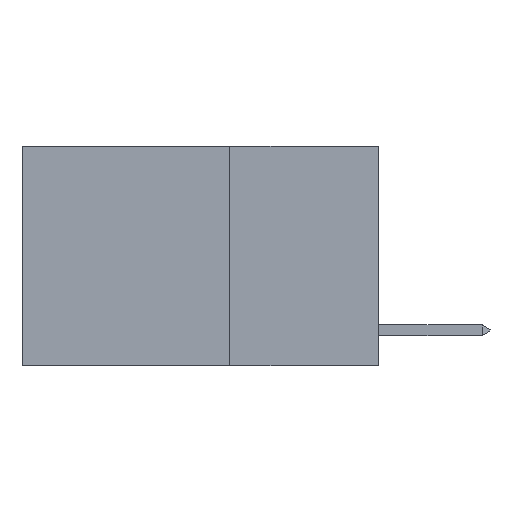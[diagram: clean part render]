
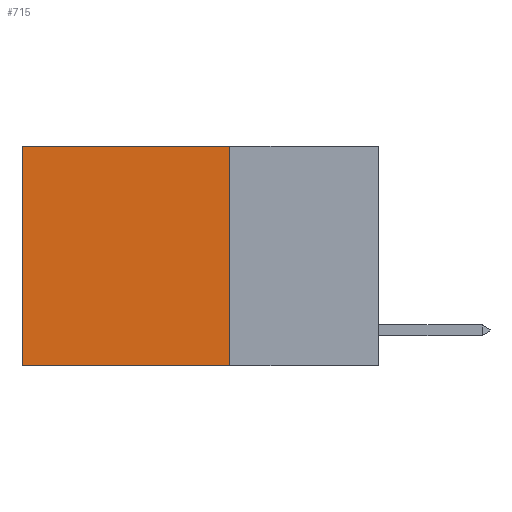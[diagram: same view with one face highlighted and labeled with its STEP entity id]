
A CAD part, left-side view. The second image highlights one B-rep face of the part: STEP entity #715.
In plain terms, the highlighted planar face has unit normal (-1, 0, 0).
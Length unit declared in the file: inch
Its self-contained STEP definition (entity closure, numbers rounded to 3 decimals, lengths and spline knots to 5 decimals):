
#715 = ADVANCED_FACE ( 'NONE', ( #7400 ), #13303, .F. ) ;
#927 = EDGE_CURVE ( 'NONE', #3811, #18361, #2249, .T. ) ;
#2249 = LINE ( 'NONE', #8657, #3781 ) ;
#3290 = LINE ( 'NONE', #7243, #19058 ) ;
#3325 = CARTESIAN_POINT ( 'NONE',  ( 0.2625, 0.25, -0.37 ) ) ;
#3564 = DIRECTION ( 'NONE',  ( 1., 0., 0. ) ) ;
#3781 = VECTOR ( 'NONE', #4310, 39.37008 ) ;
#3811 = VERTEX_POINT ( 'NONE', #4824 ) ;
#3913 = EDGE_CURVE ( 'NONE', #18361, #12568, #3290, .T. ) ;
#4310 = DIRECTION ( 'NONE',  ( 0., 1., 0. ) ) ;
#4824 = CARTESIAN_POINT ( 'NONE',  ( 0.2625, 0.25, 0. ) ) ;
#5467 = ORIENTED_EDGE ( 'NONE', *, *, #927, .T. ) ;
#7243 = CARTESIAN_POINT ( 'NONE',  ( 0.2625, 0.6, 0. ) ) ;
#7400 = FACE_OUTER_BOUND ( 'NONE', #17790, .T. ) ;
#7684 = CARTESIAN_POINT ( 'NONE',  ( 0.2625, 0.6, -0.37 ) ) ;
#8336 = EDGE_CURVE ( 'NONE', #3811, #10974, #24845, .T. ) ;
#8657 = CARTESIAN_POINT ( 'NONE',  ( 0.2625, 0.25, 0. ) ) ;
#8927 = ORIENTED_EDGE ( 'NONE', *, *, #8336, .F. ) ;
#10974 = VERTEX_POINT ( 'NONE', #3325 ) ;
#11381 = DIRECTION ( 'NONE',  ( 0., 0., -1. ) ) ;
#11484 = CARTESIAN_POINT ( 'NONE',  ( 0.2625, 0.25, 0. ) ) ;
#11681 = VECTOR ( 'NONE', #23865, 39.37008 ) ;
#11689 = ORIENTED_EDGE ( 'NONE', *, *, #14106, .F. ) ;
#12568 = VERTEX_POINT ( 'NONE', #7684 ) ;
#13303 = PLANE ( 'NONE',  #15225 ) ;
#13421 = DIRECTION ( 'NONE',  ( 0., 0., -1. ) ) ;
#14106 = EDGE_CURVE ( 'NONE', #10974, #12568, #16587, .T. ) ;
#15225 = AXIS2_PLACEMENT_3D ( 'NONE', #21033, #3564, #11381 ) ;
#16587 = LINE ( 'NONE', #20416, #11681 ) ;
#17790 = EDGE_LOOP ( 'NONE', ( #24351, #11689, #8927, #5467 ) ) ;
#18361 = VERTEX_POINT ( 'NONE', #24097 ) ;
#19058 = VECTOR ( 'NONE', #22681, 39.37008 ) ;
#20416 = CARTESIAN_POINT ( 'NONE',  ( 0.2625, 0.25, -0.37 ) ) ;
#21033 = CARTESIAN_POINT ( 'NONE',  ( 0.2625, 0.25, 0. ) ) ;
#22681 = DIRECTION ( 'NONE',  ( 0., 0., -1. ) ) ;
#22794 = VECTOR ( 'NONE', #13421, 39.37008 ) ;
#23865 = DIRECTION ( 'NONE',  ( 0., 1., 0. ) ) ;
#24097 = CARTESIAN_POINT ( 'NONE',  ( 0.2625, 0.6, 0. ) ) ;
#24351 = ORIENTED_EDGE ( 'NONE', *, *, #3913, .T. ) ;
#24845 = LINE ( 'NONE', #11484, #22794 ) ;
